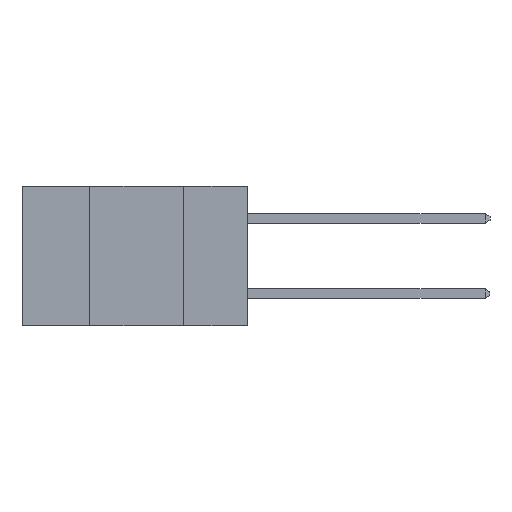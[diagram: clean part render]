
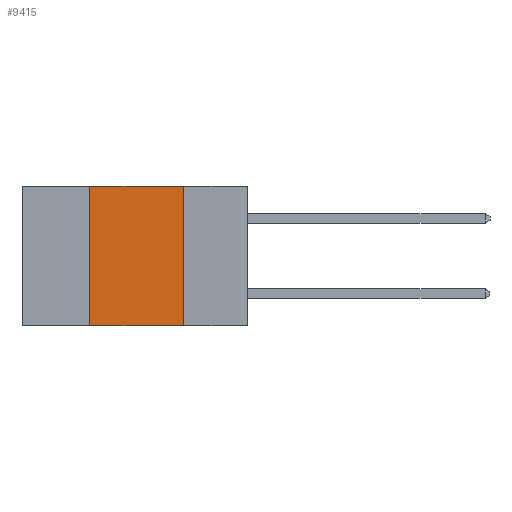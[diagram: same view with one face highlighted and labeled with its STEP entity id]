
A CAD part, left-side view. The second image highlights one B-rep face of the part: STEP entity #9415.
In plain terms, the highlighted planar face has unit normal (-1, 0, 0).
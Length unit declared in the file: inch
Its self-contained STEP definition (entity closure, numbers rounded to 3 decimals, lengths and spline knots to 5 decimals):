
#595 = PLANE ( 'NONE',  #17643 ) ;
#609 = CARTESIAN_POINT ( 'NONE',  ( 0., 0.17, 0. ) ) ;
#862 = DIRECTION ( 'NONE',  ( 0., 0., 1. ) ) ;
#2582 = VECTOR ( 'NONE', #11523, 39.37008 ) ;
#2686 = DIRECTION ( 'NONE',  ( 0., -1., 0. ) ) ;
#3967 = FACE_OUTER_BOUND ( 'NONE', #21511, .T. ) ;
#5299 = ORIENTED_EDGE ( 'NONE', *, *, #21413, .F. ) ;
#6397 = VECTOR ( 'NONE', #2686, 39.37008 ) ;
#6426 = ORIENTED_EDGE ( 'NONE', *, *, #8003, .T. ) ;
#6901 = LINE ( 'NONE', #8140, #11692 ) ;
#7967 = CARTESIAN_POINT ( 'NONE',  ( 0., 0.6, 0. ) ) ;
#8003 = EDGE_CURVE ( 'NONE', #17511, #15100, #6901, .T. ) ;
#8140 = CARTESIAN_POINT ( 'NONE',  ( 0., 0.6, -0.37 ) ) ;
#9334 = CARTESIAN_POINT ( 'NONE',  ( 0., 0.42, -0.37 ) ) ;
#9415 = ADVANCED_FACE ( 'NONE', ( #3967 ), #595, .F. ) ;
#9564 = CARTESIAN_POINT ( 'NONE',  ( 0., 0.17, -0.37 ) ) ;
#9783 = DIRECTION ( 'NONE',  ( 1., 0., 0. ) ) ;
#10266 = CARTESIAN_POINT ( 'NONE',  ( 0., 0.42, 0. ) ) ;
#10980 = VERTEX_POINT ( 'NONE', #10266 ) ;
#11523 = DIRECTION ( 'NONE',  ( 0., 0., -1. ) ) ;
#11692 = VECTOR ( 'NONE', #20845, 39.37008 ) ;
#11738 = ORIENTED_EDGE ( 'NONE', *, *, #13456, .F. ) ;
#13456 = EDGE_CURVE ( 'NONE', #10980, #16144, #16021, .T. ) ;
#13541 = CARTESIAN_POINT ( 'NONE',  ( 0., 0.6, 0. ) ) ;
#15100 = VERTEX_POINT ( 'NONE', #9564 ) ;
#16021 = LINE ( 'NONE', #13541, #6397 ) ;
#16144 = VERTEX_POINT ( 'NONE', #23278 ) ;
#17179 = CARTESIAN_POINT ( 'NONE',  ( 0., 0.42, 0. ) ) ;
#17511 = VERTEX_POINT ( 'NONE', #9334 ) ;
#17643 = AXIS2_PLACEMENT_3D ( 'NONE', #7967, #9783, #22511 ) ;
#18366 = LINE ( 'NONE', #17179, #22652 ) ;
#18740 = ORIENTED_EDGE ( 'NONE', *, *, #23382, .F. ) ;
#20785 = LINE ( 'NONE', #609, #2582 ) ;
#20845 = DIRECTION ( 'NONE',  ( 0., -1., 0. ) ) ;
#21413 = EDGE_CURVE ( 'NONE', #17511, #10980, #18366, .T. ) ;
#21511 = EDGE_LOOP ( 'NONE', ( #18740, #11738, #5299, #6426 ) ) ;
#22511 = DIRECTION ( 'NONE',  ( 0., 0., -1. ) ) ;
#22652 = VECTOR ( 'NONE', #862, 39.37008 ) ;
#23278 = CARTESIAN_POINT ( 'NONE',  ( 0., 0.17, 0. ) ) ;
#23382 = EDGE_CURVE ( 'NONE', #16144, #15100, #20785, .T. ) ;
